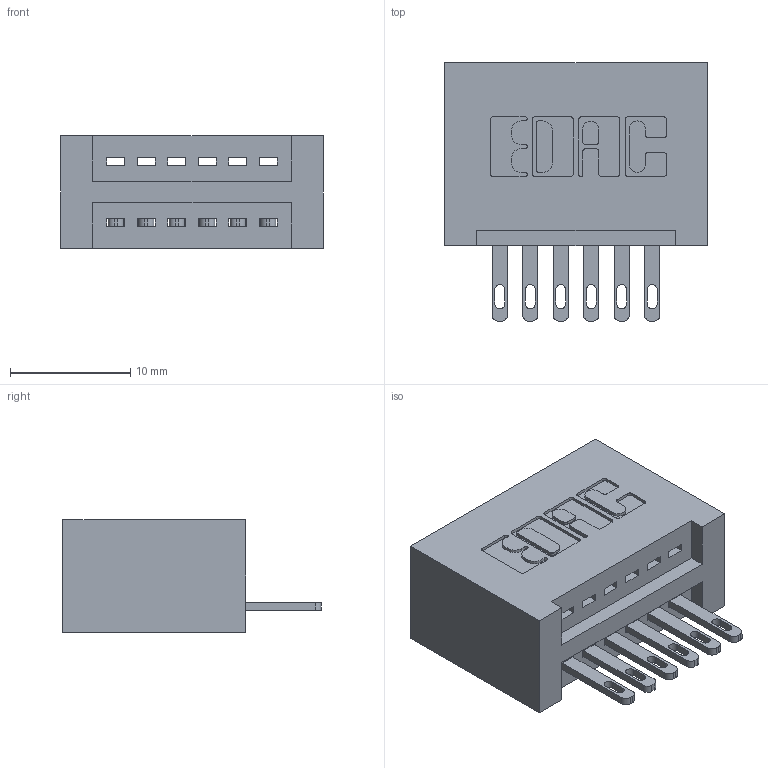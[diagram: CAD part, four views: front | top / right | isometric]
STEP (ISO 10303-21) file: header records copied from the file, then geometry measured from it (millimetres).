
FILE_DESCRIPTION (( 'STEP AP203' ), '1' );
FILE_NAME ('345-006-500-101.STEP', '2018-08-16T22:52:43', ( '' ), ( '' ), 'SwSTEP 2.0', 'SolidWorks 2016', '' );
FILE_SCHEMA (( 'CONFIG_CONTROL_DESIGN' ));
Length unit declared in the file: inch
Products named in the file (3): 345 Part_No Mounting Lugs; 345-292-001_345-293-100; 345-006-500-101
Assembly tree (7 placements, depth 2):
  345-006-500-101
    345 Part_No Mounting Lugs
    345-292-001_345-293-100  x6
Bounding box: 21.84 x 21.51 x 9.4 mm (x, y, z)
Volume: 2367.9 mm3; surface area: 2861.1 mm2
Topology: 7 solids, 7 shells, 442 faces, 1325 edges, 882 vertices
Faces by surface type: plane 280, cylinder 162
Entity records: 9015 total; most frequent: CARTESIAN_POINT 1570, ORIENTED_EDGE 1510, DIRECTION 1419, EDGE_CURVE 755, VECTOR 603, LINE 603, VERTEX_POINT 502, AXIS2_PLACEMENT_3D 408
